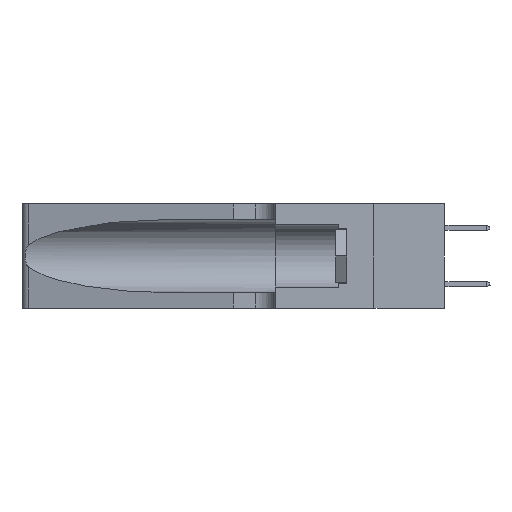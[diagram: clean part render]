
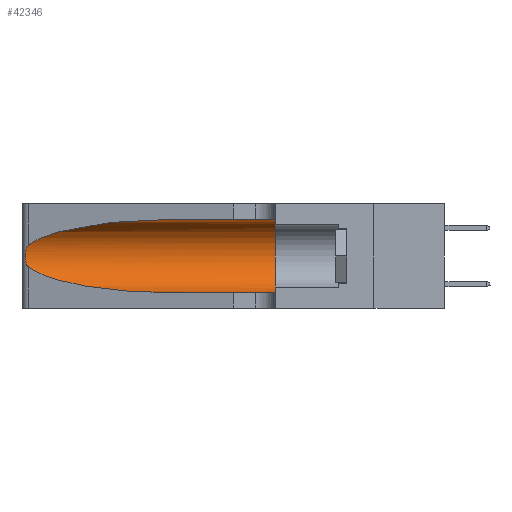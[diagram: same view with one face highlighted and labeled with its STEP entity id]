
A CAD part, left-side view. The second image highlights one B-rep face of the part: STEP entity #42346.
In plain terms, the highlighted cylindrical face has radius 3.308 mm (diameter 6.617 mm), a partial arc.
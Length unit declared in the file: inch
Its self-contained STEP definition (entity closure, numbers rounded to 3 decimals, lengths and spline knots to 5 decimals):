
#719 = CARTESIAN_POINT ( 'NONE',  ( 0.2373, 1.15595, 0.08982 ) ) ;
#1154 = CARTESIAN_POINT ( 'NONE',  ( 0.26017, 1.23833, 0.17102 ) ) ;
#1688 = CARTESIAN_POINT ( 'NONE',  ( 0.25487, 1.22718, 0.22369 ) ) ;
#1729 = ORIENTED_EDGE ( 'NONE', *, *, #3975, .T. ) ;
#1913 = CARTESIAN_POINT ( 'NONE',  ( 0.1305, 1.61858, 0.185 ) ) ;
#1976 = CYLINDRICAL_SURFACE ( 'NONE', #22354, 0.13025 ) ;
#2013 = EDGE_LOOP ( 'NONE', ( #4601, #11228, #1729, #42537, #9895, #11127 ) ) ;
#2371 = CARTESIAN_POINT ( 'NONE',  ( 0.25487, 1.22718, 0.22369 ) ) ;
#2698 = CARTESIAN_POINT ( 'NONE',  ( 0.1305, 0.72297, 0.05475 ) ) ;
#3032 = FACE_OUTER_BOUND ( 'NONE', #2013, .T. ) ;
#3607 = VERTEX_POINT ( 'NONE', #2371 ) ;
#3975 = EDGE_CURVE ( 'NONE', #13103, #41798, #40354, .T. ) ;
#4516 = CARTESIAN_POINT ( 'NONE',  ( 0.25789, 1.23486, 0.15765 ) ) ;
#4601 = ORIENTED_EDGE ( 'NONE', *, *, #12554, .T. ) ;
#5764 = EDGE_CURVE ( 'NONE', #23198, #33293, #42805, .T. ) ;
#6451 = AXIS2_PLACEMENT_3D ( 'NONE', #35903, #15704, #39254 ) ;
#7823 = CARTESIAN_POINT ( 'NONE',  ( 0.25487, 1.22718, 0.14631 ) ) ;
#7929 = CARTESIAN_POINT ( 'NONE',  ( 0.25555, 1.22993, 0.14849 ) ) ;
#7970 = VECTOR ( 'NONE', #40087, 39.37008 ) ;
#8153 = CARTESIAN_POINT ( 'NONE',  ( 0.1305, 0.35, 0.31525 ) ) ;
#8324 = CARTESIAN_POINT ( 'NONE',  ( 0.18966, 0.96281, 0.31525 ) ) ;
#8681 = DIRECTION ( 'NONE',  ( 0., -1., 0. ) ) ;
#9895 = ORIENTED_EDGE ( 'NONE', *, *, #33454, .F. ) ;
#10453 = EDGE_CURVE ( 'NONE', #3607, #13103, #24722, .T. ) ;
#10907 = CARTESIAN_POINT ( 'NONE',  ( 0.18966, 0.96281, 0.05475 ) ) ;
#11127 = ORIENTED_EDGE ( 'NONE', *, *, #5764, .F. ) ;
#11228 = ORIENTED_EDGE ( 'NONE', *, *, #10453, .T. ) ;
#11392 = CARTESIAN_POINT ( 'NONE',  ( 0.1305, 1.61858, 0.05475 ) ) ;
#12554 = EDGE_CURVE ( 'NONE', #23198, #3607, #16908, .T. ) ;
#13103 = VERTEX_POINT ( 'NONE', #7823 ) ;
#13159 = CARTESIAN_POINT ( 'NONE',  ( 0.1305, 1.61858, 0.31525 ) ) ;
#14600 = CARTESIAN_POINT ( 'NONE',  ( 0.25787, 1.23484, 0.2124 ) ) ;
#14773 = DIRECTION ( 'NONE',  ( 0., -1., 0. ) ) ;
#15704 = DIRECTION ( 'NONE',  ( 0., 1., 0. ) ) ;
#16908 =( BOUNDED_CURVE ( )  B_SPLINE_CURVE ( 3, ( #18539, #8324, #21939, #1688 ),
 .UNSPECIFIED., .F., .F. ) 
 B_SPLINE_CURVE_WITH_KNOTS ( ( 4, 4 ),
 ( 1.5708, 2.84003 ),
 .UNSPECIFIED. ) 
 CURVE ( )  GEOMETRIC_REPRESENTATION_ITEM ( )  RATIONAL_B_SPLINE_CURVE ( ( 1., 0.87, 0.87, 1. ) ) 
 REPRESENTATION_ITEM ( '' )  );
#17731 = CARTESIAN_POINT ( 'NONE',  ( 0.25487, 1.22718, 0.14631 ) ) ;
#18019 = CARTESIAN_POINT ( 'NONE',  ( 0.26018, 1.23835, 0.19895 ) ) ;
#18539 = CARTESIAN_POINT ( 'NONE',  ( 0.1305, 0.72297, 0.31525 ) ) ;
#20886 = VECTOR ( 'NONE', #14773, 39.37008 ) ;
#20963 = CARTESIAN_POINT ( 'NONE',  ( 0.25555, 1.22994, 0.2215 ) ) ;
#21108 = CARTESIAN_POINT ( 'NONE',  ( 0.1305, 0.72297, 0.05475 ) ) ;
#21395 = CARTESIAN_POINT ( 'NONE',  ( 0.26075, 1.23896, 0.178 ) ) ;
#21939 = CARTESIAN_POINT ( 'NONE',  ( 0.2373, 1.15595, 0.28018 ) ) ;
#21951 = LINE ( 'NONE', #11392, #20886 ) ;
#22354 = AXIS2_PLACEMENT_3D ( 'NONE', #1913, #8681, #32305 ) ;
#23198 = VERTEX_POINT ( 'NONE', #30878 ) ;
#23433 = CARTESIAN_POINT ( 'NONE',  ( 0.1305, 0.35, 0.05475 ) ) ;
#24722 = B_SPLINE_CURVE_WITH_KNOTS ( 'NONE', 3,
 ( #31400, #20963, #34800, #14600, #38164, #18019, #41542, #21395, #1154, #24798, #4516, #28185, #7929, #31553 ),
 .UNSPECIFIED., .F., .F.,
 ( 4, 2, 2, 2, 2, 2, 4 ),
 ( 0., 0.00027, 0.00053, 0.00107, 0.0016, 0.00187, 0.00214 ),
 .UNSPECIFIED. ) ;
#24798 = CARTESIAN_POINT ( 'NONE',  ( 0.25856, 1.23593, 0.16098 ) ) ;
#27816 = EDGE_CURVE ( 'NONE', #41798, #30890, #21951, .T. ) ;
#28185 = CARTESIAN_POINT ( 'NONE',  ( 0.25639, 1.23186, 0.15144 ) ) ;
#30878 = CARTESIAN_POINT ( 'NONE',  ( 0.1305, 0.72297, 0.31525 ) ) ;
#30890 = VERTEX_POINT ( 'NONE', #23433 ) ;
#31400 = CARTESIAN_POINT ( 'NONE',  ( 0.25487, 1.22718, 0.22369 ) ) ;
#31553 = CARTESIAN_POINT ( 'NONE',  ( 0.25487, 1.22718, 0.14631 ) ) ;
#32305 = DIRECTION ( 'NONE',  ( 0., 0., -1. ) ) ;
#33293 = VERTEX_POINT ( 'NONE', #8153 ) ;
#33454 = EDGE_CURVE ( 'NONE', #33293, #30890, #39746, .T. ) ;
#34800 = CARTESIAN_POINT ( 'NONE',  ( 0.25639, 1.23184, 0.21858 ) ) ;
#35903 = CARTESIAN_POINT ( 'NONE',  ( 0.1305, 0.35, 0.185 ) ) ;
#38164 = CARTESIAN_POINT ( 'NONE',  ( 0.25854, 1.2359, 0.20912 ) ) ;
#39254 = DIRECTION ( 'NONE',  ( 0., 0., 1. ) ) ;
#39746 = CIRCLE ( 'NONE', #6451, 0.13025 ) ;
#40087 = DIRECTION ( 'NONE',  ( 0., -1., 0. ) ) ;
#40354 =( BOUNDED_CURVE ( )  B_SPLINE_CURVE ( 3, ( #17731, #719, #10907, #21108 ),
 .UNSPECIFIED., .F., .F. ) 
 B_SPLINE_CURVE_WITH_KNOTS ( ( 4, 4 ),
 ( 3.44316, 4.71239 ),
 .UNSPECIFIED. ) 
 CURVE ( )  GEOMETRIC_REPRESENTATION_ITEM ( )  RATIONAL_B_SPLINE_CURVE ( ( 1., 0.87, 0.87, 1. ) ) 
 REPRESENTATION_ITEM ( '' )  );
#41542 = CARTESIAN_POINT ( 'NONE',  ( 0.26075, 1.23896, 0.19203 ) ) ;
#41798 = VERTEX_POINT ( 'NONE', #2698 ) ;
#42346 = ADVANCED_FACE ( 'NONE', ( #3032 ), #1976, .F. ) ;
#42537 = ORIENTED_EDGE ( 'NONE', *, *, #27816, .T. ) ;
#42805 = LINE ( 'NONE', #13159, #7970 ) ;
